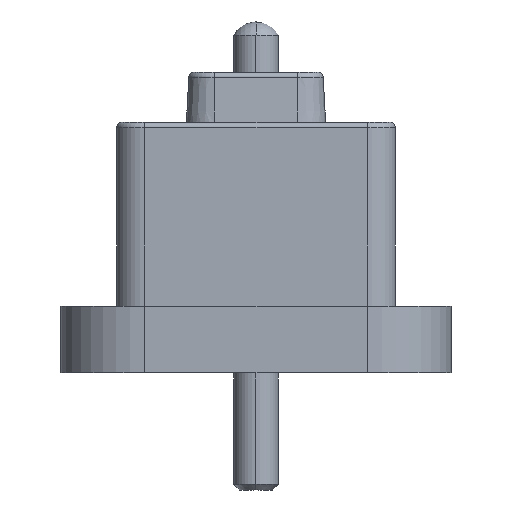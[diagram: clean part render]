
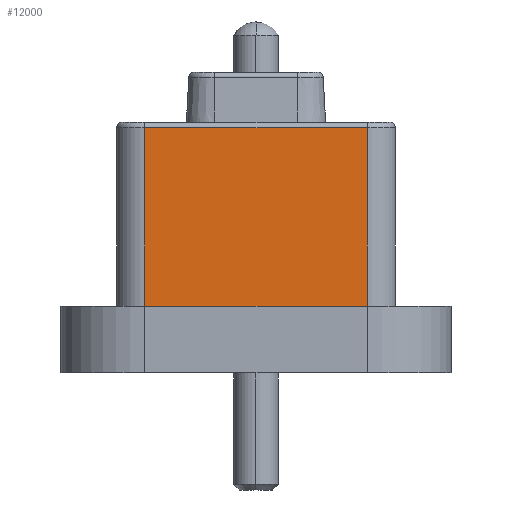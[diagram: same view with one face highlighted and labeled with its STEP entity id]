
A CAD part, left-side view. The second image highlights one B-rep face of the part: STEP entity #12000.
In plain terms, the highlighted planar face has unit normal (-1, 0, 0).
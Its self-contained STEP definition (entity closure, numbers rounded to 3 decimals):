
#479 = VECTOR ( 'NONE', #4750, 1000. ) ;
#1139 = CARTESIAN_POINT ( 'NONE',  ( -9.65, -2., -0.1 ) ) ;
#1819 = VERTEX_POINT ( 'NONE', #8084 ) ;
#2748 = LINE ( 'NONE', #7413, #10600 ) ;
#3399 = CARTESIAN_POINT ( 'NONE',  ( -9.65, 2., -0.1 ) ) ;
#3680 = LINE ( 'NONE', #7474, #479 ) ;
#3848 = EDGE_CURVE ( 'NONE', #8850, #8490, #10255, .T. ) ;
#3948 = ORIENTED_EDGE ( 'NONE', *, *, #12015, .T. ) ;
#4750 = DIRECTION ( 'NONE',  ( 0., 0., -1. ) ) ;
#4835 = EDGE_CURVE ( 'NONE', #1819, #8850, #2748, .T. ) ;
#5480 = CARTESIAN_POINT ( 'NONE',  ( -9.65, -2., -0.1 ) ) ;
#5937 = VECTOR ( 'NONE', #8097, 1000. ) ;
#6174 = ORIENTED_EDGE ( 'NONE', *, *, #3848, .T. ) ;
#6365 = VERTEX_POINT ( 'NONE', #3399 ) ;
#6418 = LINE ( 'NONE', #5480, #10642 ) ;
#6624 = DIRECTION ( 'NONE',  ( 1., 0., 0. ) ) ;
#7203 = ORIENTED_EDGE ( 'NONE', *, *, #4835, .T. ) ;
#7246 = CARTESIAN_POINT ( 'NONE',  ( -9.65, -2., -3.3 ) ) ;
#7413 = CARTESIAN_POINT ( 'NONE',  ( -9.65, 2., -3.3 ) ) ;
#7474 = CARTESIAN_POINT ( 'NONE',  ( -9.65, 2., -0.1 ) ) ;
#7483 = DIRECTION ( 'NONE',  ( 0., -1., 0. ) ) ;
#8084 = CARTESIAN_POINT ( 'NONE',  ( -9.65, 2., -3.3 ) ) ;
#8097 = DIRECTION ( 'NONE',  ( 0., 0., 1. ) ) ;
#8490 = VERTEX_POINT ( 'NONE', #1139 ) ;
#8850 = VERTEX_POINT ( 'NONE', #7246 ) ;
#9018 = CARTESIAN_POINT ( 'NONE',  ( -9.65, -2., -3.3 ) ) ;
#9344 = EDGE_LOOP ( 'NONE', ( #12035, #7203, #6174, #3948 ) ) ;
#9439 = DIRECTION ( 'NONE',  ( 0., 1., 0. ) ) ;
#10128 = DIRECTION ( 'NONE',  ( 0., 1., 0. ) ) ;
#10255 = LINE ( 'NONE', #9018, #5937 ) ;
#10524 = PLANE ( 'NONE',  #11044 ) ;
#10600 = VECTOR ( 'NONE', #7483, 1000. ) ;
#10642 = VECTOR ( 'NONE', #10128, 1000. ) ;
#11044 = AXIS2_PLACEMENT_3D ( 'NONE', #11615, #6624, #9439 ) ;
#11504 = FACE_OUTER_BOUND ( 'NONE', #9344, .T. ) ;
#11615 = CARTESIAN_POINT ( 'NONE',  ( -9.65, 0., -1.7 ) ) ;
#12000 = ADVANCED_FACE ( 'NONE', ( #11504 ), #10524, .F. ) ;
#12015 = EDGE_CURVE ( 'NONE', #8490, #6365, #6418, .T. ) ;
#12035 = ORIENTED_EDGE ( 'NONE', *, *, #12091, .T. ) ;
#12091 = EDGE_CURVE ( 'NONE', #6365, #1819, #3680, .T. ) ;
